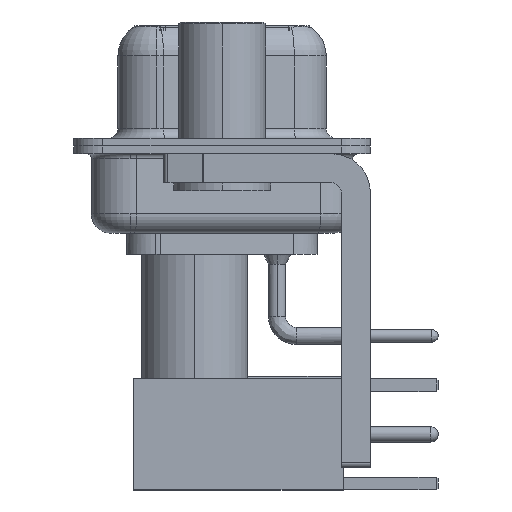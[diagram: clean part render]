
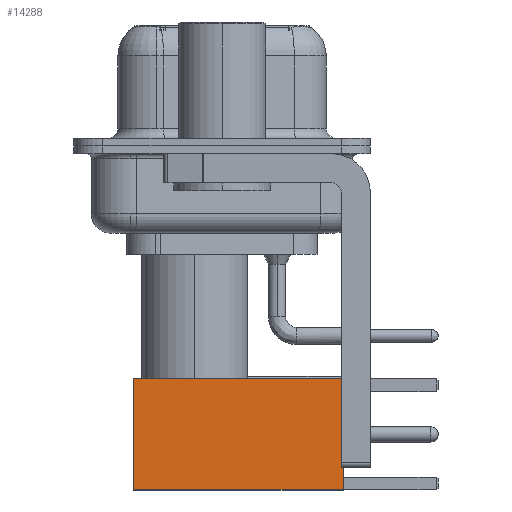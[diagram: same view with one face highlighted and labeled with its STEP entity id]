
A CAD part, left-side view. The second image highlights one B-rep face of the part: STEP entity #14288.
In plain terms, the highlighted face is planar.
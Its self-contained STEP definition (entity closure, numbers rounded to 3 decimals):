
#426 = ORIENTED_EDGE ( 'NONE', *, *, #7431, .F. ) ;
#526 = VECTOR ( 'NONE', #25544, 1000. ) ;
#2031 = LINE ( 'NONE', #13839, #34637 ) ;
#3431 = VERTEX_POINT ( 'NONE', #15903 ) ;
#5796 = LINE ( 'NONE', #18023, #33244 ) ;
#7307 = CARTESIAN_POINT ( 'NONE',  ( -2.875, 2.875, 0. ) ) ;
#7431 = EDGE_CURVE ( 'NONE', #3431, #12221, #15758, .T. ) ;
#7813 = CARTESIAN_POINT ( 'NONE',  ( -2.875, 2.875, 0. ) ) ;
#7898 = LINE ( 'NONE', #7307, #526 ) ;
#8731 = EDGE_CURVE ( 'NONE', #3431, #13798, #2031, .T. ) ;
#12221 = VERTEX_POINT ( 'NONE', #17041 ) ;
#13798 = VERTEX_POINT ( 'NONE', #25586 ) ;
#13839 = CARTESIAN_POINT ( 'NONE',  ( 2.875, 2.875, 0. ) ) ;
#13881 = EDGE_LOOP ( 'NONE', ( #15576, #16348, #14213, #426 ) ) ;
#14213 = ORIENTED_EDGE ( 'NONE', *, *, #20270, .F. ) ;
#14288 = ADVANCED_FACE ( 'NONE', ( #28161 ), #25141, .T. ) ;
#15576 = ORIENTED_EDGE ( 'NONE', *, *, #8731, .T. ) ;
#15758 = LINE ( 'NONE', #24965, #16653 ) ;
#15903 = CARTESIAN_POINT ( 'NONE',  ( 2.875, 2.875, 10.82 ) ) ;
#16348 = ORIENTED_EDGE ( 'NONE', *, *, #37436, .T. ) ;
#16653 = VECTOR ( 'NONE', #33800, 1000. ) ;
#17041 = CARTESIAN_POINT ( 'NONE',  ( -2.875, 2.875, 10.82 ) ) ;
#18023 = CARTESIAN_POINT ( 'NONE',  ( 0., 2.875, 0. ) ) ;
#20270 = EDGE_CURVE ( 'NONE', #12221, #28776, #7898, .T. ) ;
#23043 = DIRECTION ( 'NONE',  ( 0., 0., -1. ) ) ;
#24609 = AXIS2_PLACEMENT_3D ( 'NONE', #30988, #34176, #36796 ) ;
#24965 = CARTESIAN_POINT ( 'NONE',  ( 0., 2.875, 10.82 ) ) ;
#25141 = PLANE ( 'NONE',  #24609 ) ;
#25544 = DIRECTION ( 'NONE',  ( 0., 0., -1. ) ) ;
#25586 = CARTESIAN_POINT ( 'NONE',  ( 2.875, 2.875, 0. ) ) ;
#28161 = FACE_OUTER_BOUND ( 'NONE', #13881, .T. ) ;
#28776 = VERTEX_POINT ( 'NONE', #7813 ) ;
#30240 = DIRECTION ( 'NONE',  ( -1., 0., 0. ) ) ;
#30988 = CARTESIAN_POINT ( 'NONE',  ( 2.875, 2.875, 0. ) ) ;
#33244 = VECTOR ( 'NONE', #30240, 1000. ) ;
#33800 = DIRECTION ( 'NONE',  ( -1., 0., 0. ) ) ;
#34176 = DIRECTION ( 'NONE',  ( 0., 1., 0. ) ) ;
#34637 = VECTOR ( 'NONE', #23043, 1000. ) ;
#36796 = DIRECTION ( 'NONE',  ( 0., 0., 1. ) ) ;
#37436 = EDGE_CURVE ( 'NONE', #13798, #28776, #5796, .T. ) ;
